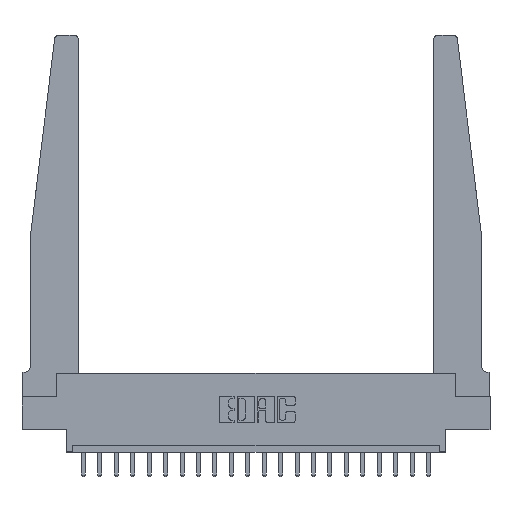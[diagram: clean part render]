
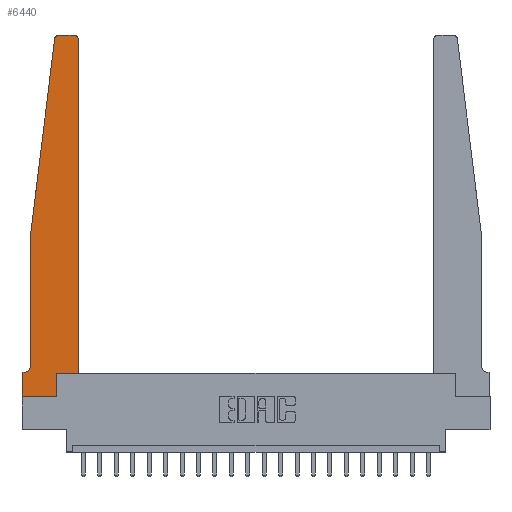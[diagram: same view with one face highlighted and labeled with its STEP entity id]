
A CAD part, top view. The second image highlights one B-rep face of the part: STEP entity #6440.
In plain terms, the highlighted planar face has unit normal (0, 0, 1).
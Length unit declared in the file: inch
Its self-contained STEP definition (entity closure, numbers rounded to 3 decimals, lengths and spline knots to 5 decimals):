
#102 = LINE ( 'NONE', #15189, #18161 ) ;
#117 = EDGE_CURVE ( 'NONE', #6600, #8722, #159, .T. ) ;
#159 = LINE ( 'NONE', #14872, #17172 ) ;
#400 = ORIENTED_EDGE ( 'NONE', *, *, #18333, .T. ) ;
#656 = EDGE_CURVE ( 'NONE', #16649, #11061, #15831, .T. ) ;
#1176 = CARTESIAN_POINT ( 'NONE',  ( 0., 0., 0.37 ) ) ;
#1236 = LINE ( 'NONE', #19878, #21093 ) ;
#1416 = VECTOR ( 'NONE', #9460, 39.37008 ) ;
#1528 = VECTOR ( 'NONE', #4181, 39.37008 ) ;
#1733 = CARTESIAN_POINT ( 'NONE',  ( 0.065, 1.25, 0.37 ) ) ;
#1736 = EDGE_CURVE ( 'NONE', #15359, #17268, #8835, .T. ) ;
#1990 = EDGE_CURVE ( 'NONE', #5921, #7392, #102, .T. ) ;
#2044 = DIRECTION ( 'NONE',  ( 0., 0., 1. ) ) ;
#2096 = CARTESIAN_POINT ( 'NONE',  ( 0.25, 2.75, 0.37 ) ) ;
#2548 = AXIS2_PLACEMENT_3D ( 'NONE', #19874, #8508, #6557 ) ;
#3176 = EDGE_CURVE ( 'NONE', #9465, #5921, #4919, .T. ) ;
#3613 = PLANE ( 'NONE',  #9571 ) ;
#3821 = ORIENTED_EDGE ( 'NONE', *, *, #8578, .T. ) ;
#4113 = CARTESIAN_POINT ( 'NONE',  ( 0.27653, 2.75, 0.37 ) ) ;
#4181 = DIRECTION ( 'NONE',  ( 0., 1., 0. ) ) ;
#4325 = LINE ( 'NONE', #17643, #13833 ) ;
#4669 = VECTOR ( 'NONE', #13205, 39.37008 ) ;
#4919 = CIRCLE ( 'NONE', #14118, 0.03 ) ;
#4924 = DIRECTION ( 'NONE',  ( 0., 1., 0. ) ) ;
#5089 = LINE ( 'NONE', #12361, #1528 ) ;
#5515 = VECTOR ( 'NONE', #19024, 39.37008 ) ;
#5921 = VERTEX_POINT ( 'NONE', #19340 ) ;
#6124 = VERTEX_POINT ( 'NONE', #8982 ) ;
#6300 = DIRECTION ( 'NONE',  ( -1., 0., 0. ) ) ;
#6440 = ADVANCED_FACE ( 'NONE', ( #13341 ), #3613, .T. ) ;
#6557 = DIRECTION ( 'NONE',  ( -1., 0., 0. ) ) ;
#6600 = VERTEX_POINT ( 'NONE', #13562 ) ;
#6656 = EDGE_CURVE ( 'NONE', #7770, #15359, #4325, .T. ) ;
#6789 = ORIENTED_EDGE ( 'NONE', *, *, #3176, .T. ) ;
#6984 = CIRCLE ( 'NONE', #2548, 0.05 ) ;
#7096 = DIRECTION ( 'NONE',  ( -1., 0., 0. ) ) ;
#7209 = CARTESIAN_POINT ( 'NONE',  ( 0.425, 0.18, 0.37 ) ) ;
#7356 = DIRECTION ( 'NONE',  ( 1., 0., 0. ) ) ;
#7392 = VERTEX_POINT ( 'NONE', #17763 ) ;
#7751 = DIRECTION ( 'NONE',  ( 0., 0., 1. ) ) ;
#7770 = VERTEX_POINT ( 'NONE', #20300 ) ;
#7828 = ORIENTED_EDGE ( 'NONE', *, *, #1736, .T. ) ;
#8508 = DIRECTION ( 'NONE',  ( 0., 0., -1. ) ) ;
#8578 = EDGE_CURVE ( 'NONE', #11061, #9465, #16381, .T. ) ;
#8648 = EDGE_LOOP ( 'NONE', ( #3821, #6789, #18567, #15182, #19295, #10101, #7828, #11136, #400, #11303, #11861, #11250 ) ) ;
#8722 = VERTEX_POINT ( 'NONE', #7209 ) ;
#8835 = LINE ( 'NONE', #1176, #1416 ) ;
#8982 = CARTESIAN_POINT ( 'NONE',  ( 0.2605, 0., 0.37 ) ) ;
#9447 = VERTEX_POINT ( 'NONE', #13660 ) ;
#9460 = DIRECTION ( 'NONE',  ( 0., -1., 0. ) ) ;
#9465 = VERTEX_POINT ( 'NONE', #4113 ) ;
#9571 = AXIS2_PLACEMENT_3D ( 'NONE', #16720, #2044, #13519 ) ;
#9767 = CARTESIAN_POINT ( 'NONE',  ( 0.395, 2.75, 0.37 ) ) ;
#10101 = ORIENTED_EDGE ( 'NONE', *, *, #6656, .T. ) ;
#10661 = DIRECTION ( 'NONE',  ( 0., 0., 1. ) ) ;
#11061 = VERTEX_POINT ( 'NONE', #9767 ) ;
#11136 = ORIENTED_EDGE ( 'NONE', *, *, #17618, .T. ) ;
#11250 = ORIENTED_EDGE ( 'NONE', *, *, #656, .T. ) ;
#11303 = ORIENTED_EDGE ( 'NONE', *, *, #117, .T. ) ;
#11421 = LINE ( 'NONE', #12049, #5515 ) ;
#11851 = DIRECTION ( 'NONE',  ( -0.122, -0.992, 0. ) ) ;
#11861 = ORIENTED_EDGE ( 'NONE', *, *, #19144, .T. ) ;
#12049 = CARTESIAN_POINT ( 'NONE',  ( 0., 0., 0.37 ) ) ;
#12361 = CARTESIAN_POINT ( 'NONE',  ( 0.2605, 0.18, 0.37 ) ) ;
#12845 = AXIS2_PLACEMENT_3D ( 'NONE', #16210, #7751, #19360 ) ;
#12902 = EDGE_CURVE ( 'NONE', #9447, #7770, #6984, .T. ) ;
#13066 = EDGE_CURVE ( 'NONE', #7392, #9447, #13419, .T. ) ;
#13205 = DIRECTION ( 'NONE',  ( 0., -1., 0. ) ) ;
#13255 = VECTOR ( 'NONE', #7096, 39.37008 ) ;
#13341 = FACE_OUTER_BOUND ( 'NONE', #8648, .T. ) ;
#13419 = LINE ( 'NONE', #1733, #4669 ) ;
#13519 = DIRECTION ( 'NONE',  ( 1., 0., 0. ) ) ;
#13562 = CARTESIAN_POINT ( 'NONE',  ( 0.2605, 0.18, 0.37 ) ) ;
#13660 = CARTESIAN_POINT ( 'NONE',  ( 0.065, 0.2375, 0.37 ) ) ;
#13833 = VECTOR ( 'NONE', #6300, 39.37008 ) ;
#14118 = AXIS2_PLACEMENT_3D ( 'NONE', #15597, #10661, #7356 ) ;
#14872 = CARTESIAN_POINT ( 'NONE',  ( 0.425, 0.18, 0.37 ) ) ;
#15182 = ORIENTED_EDGE ( 'NONE', *, *, #13066, .T. ) ;
#15189 = CARTESIAN_POINT ( 'NONE',  ( 0.065, 1.25, 0.37 ) ) ;
#15359 = VERTEX_POINT ( 'NONE', #17784 ) ;
#15597 = CARTESIAN_POINT ( 'NONE',  ( 0.27653, 2.72, 0.37 ) ) ;
#15831 = CIRCLE ( 'NONE', #12845, 0.03 ) ;
#16210 = CARTESIAN_POINT ( 'NONE',  ( 0.395, 2.72, 0.37 ) ) ;
#16381 = LINE ( 'NONE', #2096, #13255 ) ;
#16649 = VERTEX_POINT ( 'NONE', #17446 ) ;
#16720 = CARTESIAN_POINT ( 'NONE',  ( 0., 0.1875, 0.37 ) ) ;
#17172 = VECTOR ( 'NONE', #19583, 39.37008 ) ;
#17268 = VERTEX_POINT ( 'NONE', #18823 ) ;
#17446 = CARTESIAN_POINT ( 'NONE',  ( 0.425, 2.72, 0.37 ) ) ;
#17618 = EDGE_CURVE ( 'NONE', #17268, #6124, #11421, .T. ) ;
#17643 = CARTESIAN_POINT ( 'NONE',  ( 0.065, 0.1875, 0.37 ) ) ;
#17763 = CARTESIAN_POINT ( 'NONE',  ( 0.065, 1.25, 0.37 ) ) ;
#17784 = CARTESIAN_POINT ( 'NONE',  ( 0., 0.1875, 0.37 ) ) ;
#18161 = VECTOR ( 'NONE', #11851, 39.37008 ) ;
#18333 = EDGE_CURVE ( 'NONE', #6124, #6600, #5089, .T. ) ;
#18567 = ORIENTED_EDGE ( 'NONE', *, *, #1990, .T. ) ;
#18823 = CARTESIAN_POINT ( 'NONE',  ( 0., 0., 0.37 ) ) ;
#19024 = DIRECTION ( 'NONE',  ( 1., 0., 0. ) ) ;
#19144 = EDGE_CURVE ( 'NONE', #8722, #16649, #1236, .T. ) ;
#19295 = ORIENTED_EDGE ( 'NONE', *, *, #12902, .T. ) ;
#19340 = CARTESIAN_POINT ( 'NONE',  ( 0.24675, 2.72367, 0.37 ) ) ;
#19360 = DIRECTION ( 'NONE',  ( 1., 0., 0. ) ) ;
#19583 = DIRECTION ( 'NONE',  ( 1., 0., 0. ) ) ;
#19874 = CARTESIAN_POINT ( 'NONE',  ( 0.015, 0.2375, 0.37 ) ) ;
#19878 = CARTESIAN_POINT ( 'NONE',  ( 0.425, 0.18, 0.37 ) ) ;
#20300 = CARTESIAN_POINT ( 'NONE',  ( 0.015, 0.1875, 0.37 ) ) ;
#21093 = VECTOR ( 'NONE', #4924, 39.37008 ) ;
